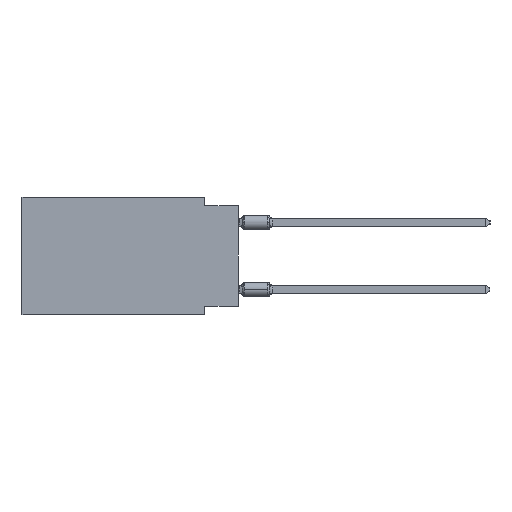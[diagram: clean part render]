
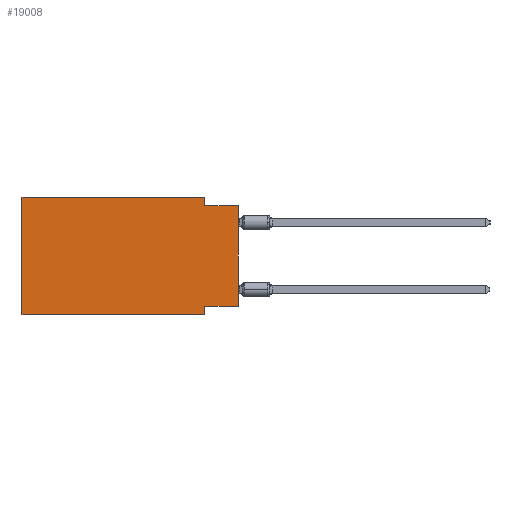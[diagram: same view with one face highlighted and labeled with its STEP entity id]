
A CAD part, left-side view. The second image highlights one B-rep face of the part: STEP entity #19008.
In plain terms, the highlighted planar face has unit normal (-1, 0, 0).
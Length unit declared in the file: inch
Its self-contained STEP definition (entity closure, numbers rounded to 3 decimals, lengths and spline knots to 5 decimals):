
#297 = VERTEX_POINT ( 'NONE', #24122 ) ;
#1109 = EDGE_CURVE ( 'NONE', #2757, #8728, #20763, .T. ) ;
#2757 = VERTEX_POINT ( 'NONE', #35046 ) ;
#3754 = DIRECTION ( 'NONE',  ( 0., 0., 1. ) ) ;
#3962 = EDGE_CURVE ( 'NONE', #17689, #21490, #6029, .T. ) ;
#6029 = LINE ( 'NONE', #32208, #27886 ) ;
#6042 = DIRECTION ( 'NONE',  ( 0., 0., -1. ) ) ;
#6513 = EDGE_CURVE ( 'NONE', #37686, #17689, #28584, .T. ) ;
#6538 = VECTOR ( 'NONE', #28631, 39.37008 ) ;
#7530 = DIRECTION ( 'NONE',  ( 0., 0., -1. ) ) ;
#8325 = EDGE_LOOP ( 'NONE', ( #19471, #26321, #38614, #41202, #33699, #40074, #12366, #9677 ) ) ;
#8728 = VERTEX_POINT ( 'NONE', #25970 ) ;
#8810 = VECTOR ( 'NONE', #16780, 39.37008 ) ;
#9023 = CARTESIAN_POINT ( 'NONE',  ( 0., 0., -0.325 ) ) ;
#9298 = VERTEX_POINT ( 'NONE', #39129 ) ;
#9677 = ORIENTED_EDGE ( 'NONE', *, *, #25250, .F. ) ;
#10793 = LINE ( 'NONE', #13356, #20183 ) ;
#12366 = ORIENTED_EDGE ( 'NONE', *, *, #13055, .F. ) ;
#13055 = EDGE_CURVE ( 'NONE', #9298, #36174, #40943, .T. ) ;
#13356 = CARTESIAN_POINT ( 'NONE',  ( 0., 0., 0. ) ) ;
#13513 = CARTESIAN_POINT ( 'NONE',  ( 0., 0.645, 0. ) ) ;
#14376 = CARTESIAN_POINT ( 'NONE',  ( 0., 0.645, 0. ) ) ;
#14762 = DIRECTION ( 'NONE',  ( 0., 0., -1. ) ) ;
#15440 = CARTESIAN_POINT ( 'NONE',  ( 0., 0.1, -0.35 ) ) ;
#16144 = VECTOR ( 'NONE', #6042, 39.37008 ) ;
#16671 = PLANE ( 'NONE',  #21510 ) ;
#16780 = DIRECTION ( 'NONE',  ( 0., 0., 1. ) ) ;
#17689 = VERTEX_POINT ( 'NONE', #14376 ) ;
#18242 = LINE ( 'NONE', #9023, #6538 ) ;
#19008 = ADVANCED_FACE ( 'NONE', ( #32868 ), #16671, .F. ) ;
#19011 = DIRECTION ( 'NONE',  ( 0., -1., 0. ) ) ;
#19471 = ORIENTED_EDGE ( 'NONE', *, *, #20309, .T. ) ;
#19791 = CARTESIAN_POINT ( 'NONE',  ( 0., 0.1, 0. ) ) ;
#20183 = VECTOR ( 'NONE', #3754, 39.37008 ) ;
#20309 = EDGE_CURVE ( 'NONE', #297, #8728, #10793, .T. ) ;
#20763 = LINE ( 'NONE', #23309, #24109 ) ;
#21490 = VERTEX_POINT ( 'NONE', #19791 ) ;
#21510 = AXIS2_PLACEMENT_3D ( 'NONE', #13513, #26488, #7530 ) ;
#22017 = LINE ( 'NONE', #38375, #36253 ) ;
#22405 = CARTESIAN_POINT ( 'NONE',  ( 0., 0.645, 0. ) ) ;
#22410 = EDGE_CURVE ( 'NONE', #21490, #2757, #34118, .T. ) ;
#23309 = CARTESIAN_POINT ( 'NONE',  ( 0., 0., -0.025 ) ) ;
#24109 = VECTOR ( 'NONE', #26695, 39.37008 ) ;
#24122 = CARTESIAN_POINT ( 'NONE',  ( 0., 0., -0.325 ) ) ;
#25250 = EDGE_CURVE ( 'NONE', #297, #9298, #18242, .T. ) ;
#25970 = CARTESIAN_POINT ( 'NONE',  ( 0., 0., -0.025 ) ) ;
#26321 = ORIENTED_EDGE ( 'NONE', *, *, #1109, .F. ) ;
#26488 = DIRECTION ( 'NONE',  ( 1., 0., 0. ) ) ;
#26695 = DIRECTION ( 'NONE',  ( 0., -1., 0. ) ) ;
#27886 = VECTOR ( 'NONE', #19011, 39.37008 ) ;
#28584 = LINE ( 'NONE', #22405, #8810 ) ;
#28631 = DIRECTION ( 'NONE',  ( 0., 1., 0. ) ) ;
#28816 = DIRECTION ( 'NONE',  ( 0., -1., 0. ) ) ;
#29101 = EDGE_CURVE ( 'NONE', #37686, #36174, #22017, .T. ) ;
#29550 = CARTESIAN_POINT ( 'NONE',  ( 0., 0.645, -0.35 ) ) ;
#31163 = CARTESIAN_POINT ( 'NONE',  ( 0., 0.1, 0. ) ) ;
#31940 = CARTESIAN_POINT ( 'NONE',  ( 0., 0.1, -0.35 ) ) ;
#32208 = CARTESIAN_POINT ( 'NONE',  ( 0., 0.645, 0. ) ) ;
#32868 = FACE_OUTER_BOUND ( 'NONE', #8325, .T. ) ;
#33699 = ORIENTED_EDGE ( 'NONE', *, *, #6513, .F. ) ;
#34118 = LINE ( 'NONE', #31163, #41024 ) ;
#35046 = CARTESIAN_POINT ( 'NONE',  ( 0., 0.1, -0.025 ) ) ;
#36174 = VERTEX_POINT ( 'NONE', #31940 ) ;
#36253 = VECTOR ( 'NONE', #28816, 39.37008 ) ;
#37686 = VERTEX_POINT ( 'NONE', #29550 ) ;
#38375 = CARTESIAN_POINT ( 'NONE',  ( 0., 0.645, -0.35 ) ) ;
#38614 = ORIENTED_EDGE ( 'NONE', *, *, #22410, .F. ) ;
#39129 = CARTESIAN_POINT ( 'NONE',  ( 0., 0.1, -0.325 ) ) ;
#40074 = ORIENTED_EDGE ( 'NONE', *, *, #29101, .T. ) ;
#40943 = LINE ( 'NONE', #15440, #16144 ) ;
#41024 = VECTOR ( 'NONE', #14762, 39.37008 ) ;
#41202 = ORIENTED_EDGE ( 'NONE', *, *, #3962, .F. ) ;
